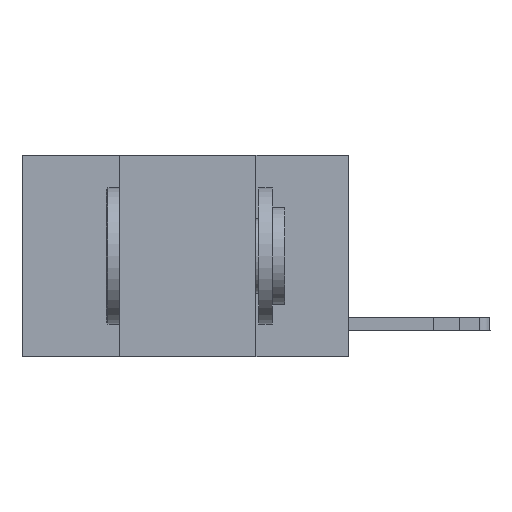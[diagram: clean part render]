
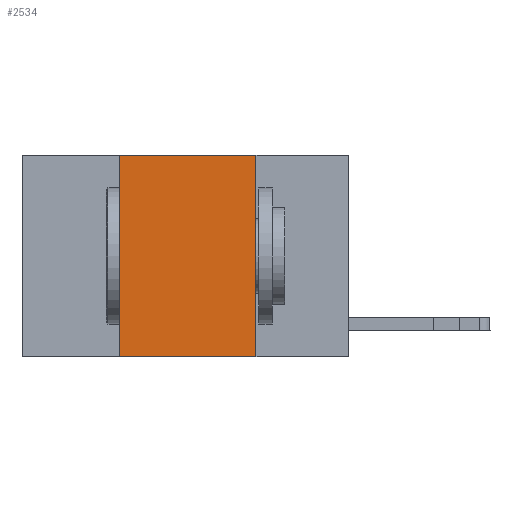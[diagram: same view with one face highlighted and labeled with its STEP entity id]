
A CAD part, left-side view. The second image highlights one B-rep face of the part: STEP entity #2534.
In plain terms, the highlighted planar face has unit normal (-1, 0, 0).
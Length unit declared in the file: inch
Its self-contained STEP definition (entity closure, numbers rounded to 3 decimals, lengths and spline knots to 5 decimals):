
#210 = DIRECTION ( 'NONE',  ( 0., -1., 0. ) ) ;
#1344 = ORIENTED_EDGE ( 'NONE', *, *, #6112, .F. ) ;
#2534 = ADVANCED_FACE ( 'NONE', ( #21364 ), #7885, .F. ) ;
#3112 = CARTESIAN_POINT ( 'NONE',  ( 0., 0.6, -0.37 ) ) ;
#3402 = CARTESIAN_POINT ( 'NONE',  ( 0., 0.17, -0.37 ) ) ;
#4262 = VECTOR ( 'NONE', #18018, 39.37008 ) ;
#5216 = LINE ( 'NONE', #10402, #9276 ) ;
#5393 = EDGE_CURVE ( 'NONE', #16266, #9392, #12413, .T. ) ;
#5686 = CARTESIAN_POINT ( 'NONE',  ( 0., 0.42, 0. ) ) ;
#6112 = EDGE_CURVE ( 'NONE', #9392, #8371, #5216, .T. ) ;
#6246 = CARTESIAN_POINT ( 'NONE',  ( 0., 0.42, -0.37 ) ) ;
#6403 = CARTESIAN_POINT ( 'NONE',  ( 0., 0.42, 0. ) ) ;
#6644 = ORIENTED_EDGE ( 'NONE', *, *, #17645, .F. ) ;
#6664 = AXIS2_PLACEMENT_3D ( 'NONE', #14495, #14724, #9749 ) ;
#7716 = EDGE_CURVE ( 'NONE', #16266, #13896, #21666, .T. ) ;
#7885 = PLANE ( 'NONE',  #6664 ) ;
#8371 = VERTEX_POINT ( 'NONE', #15444 ) ;
#9276 = VECTOR ( 'NONE', #210, 39.37008 ) ;
#9392 = VERTEX_POINT ( 'NONE', #6403 ) ;
#9749 = DIRECTION ( 'NONE',  ( 0., 0., -1. ) ) ;
#10402 = CARTESIAN_POINT ( 'NONE',  ( 0., 0.6, 0. ) ) ;
#11088 = DIRECTION ( 'NONE',  ( 0., 0., -1. ) ) ;
#11425 = LINE ( 'NONE', #16523, #11828 ) ;
#11828 = VECTOR ( 'NONE', #11088, 39.37008 ) ;
#12413 = LINE ( 'NONE', #5686, #13908 ) ;
#13896 = VERTEX_POINT ( 'NONE', #3402 ) ;
#13908 = VECTOR ( 'NONE', #19163, 39.37008 ) ;
#14495 = CARTESIAN_POINT ( 'NONE',  ( 0., 0.6, 0. ) ) ;
#14724 = DIRECTION ( 'NONE',  ( 1., 0., 0. ) ) ;
#15444 = CARTESIAN_POINT ( 'NONE',  ( 0., 0.17, 0. ) ) ;
#16266 = VERTEX_POINT ( 'NONE', #6246 ) ;
#16523 = CARTESIAN_POINT ( 'NONE',  ( 0., 0.17, 0. ) ) ;
#17645 = EDGE_CURVE ( 'NONE', #8371, #13896, #11425, .T. ) ;
#18018 = DIRECTION ( 'NONE',  ( 0., -1., 0. ) ) ;
#18231 = ORIENTED_EDGE ( 'NONE', *, *, #7716, .T. ) ;
#18813 = ORIENTED_EDGE ( 'NONE', *, *, #5393, .F. ) ;
#19163 = DIRECTION ( 'NONE',  ( 0., 0., 1. ) ) ;
#20796 = EDGE_LOOP ( 'NONE', ( #6644, #1344, #18813, #18231 ) ) ;
#21364 = FACE_OUTER_BOUND ( 'NONE', #20796, .T. ) ;
#21666 = LINE ( 'NONE', #3112, #4262 ) ;
